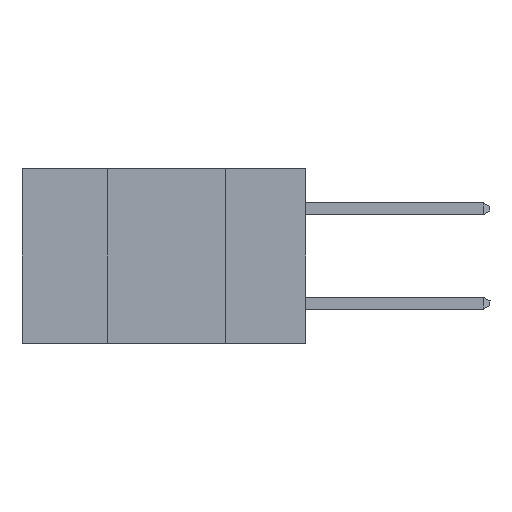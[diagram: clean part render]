
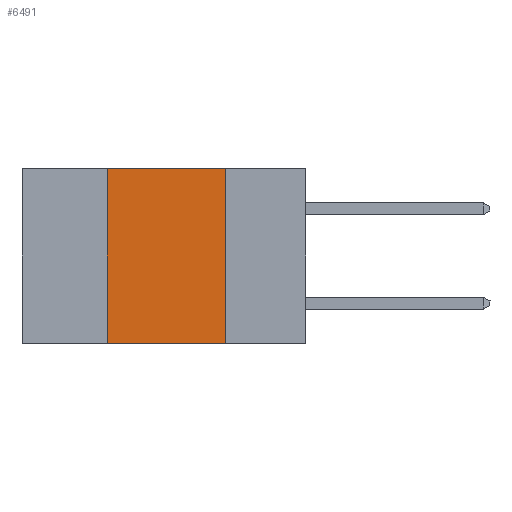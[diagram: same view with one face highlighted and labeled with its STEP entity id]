
A CAD part, left-side view. The second image highlights one B-rep face of the part: STEP entity #6491.
In plain terms, the highlighted planar face has unit normal (-1, 0, 0).
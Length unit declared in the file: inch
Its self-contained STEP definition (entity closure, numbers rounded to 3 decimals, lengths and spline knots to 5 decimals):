
#111 = VECTOR ( 'NONE', #6133, 39.37008 ) ;
#2327 = VECTOR ( 'NONE', #5412, 39.37008 ) ;
#3230 = LINE ( 'NONE', #7693, #8571 ) ;
#3792 = ORIENTED_EDGE ( 'NONE', *, *, #4248, .F. ) ;
#3851 = VERTEX_POINT ( 'NONE', #7272 ) ;
#3868 = ORIENTED_EDGE ( 'NONE', *, *, #4463, .F. ) ;
#4248 = EDGE_CURVE ( 'NONE', #3851, #10969, #10044, .T. ) ;
#4463 = EDGE_CURVE ( 'NONE', #10969, #12959, #3230, .T. ) ;
#5000 = EDGE_CURVE ( 'NONE', #13217, #12959, #14022, .T. ) ;
#5136 = CARTESIAN_POINT ( 'NONE',  ( 0., 0.6, 0. ) ) ;
#5210 = EDGE_CURVE ( 'NONE', #13217, #3851, #12426, .T. ) ;
#5412 = DIRECTION ( 'NONE',  ( 0., -1., 0. ) ) ;
#6133 = DIRECTION ( 'NONE',  ( 0., 0., 1. ) ) ;
#6328 = ORIENTED_EDGE ( 'NONE', *, *, #5000, .T. ) ;
#6337 = FACE_OUTER_BOUND ( 'NONE', #12297, .T. ) ;
#6429 = DIRECTION ( 'NONE',  ( 0., 0., -1. ) ) ;
#6491 = ADVANCED_FACE ( 'NONE', ( #6337 ), #8418, .F. ) ;
#6568 = DIRECTION ( 'NONE',  ( 0., 0., -1. ) ) ;
#6852 = CARTESIAN_POINT ( 'NONE',  ( 0., 0.17, -0.37 ) ) ;
#6956 = CARTESIAN_POINT ( 'NONE',  ( 0., 0.6, -0.37 ) ) ;
#7272 = CARTESIAN_POINT ( 'NONE',  ( 0., 0.42, 0. ) ) ;
#7686 = CARTESIAN_POINT ( 'NONE',  ( 0., 0.17, 0. ) ) ;
#7693 = CARTESIAN_POINT ( 'NONE',  ( 0., 0.17, 0. ) ) ;
#8418 = PLANE ( 'NONE',  #11963 ) ;
#8571 = VECTOR ( 'NONE', #6568, 39.37008 ) ;
#8695 = DIRECTION ( 'NONE',  ( 1., 0., 0. ) ) ;
#10044 = LINE ( 'NONE', #14464, #2327 ) ;
#10214 = CARTESIAN_POINT ( 'NONE',  ( 0., 0.42, -0.37 ) ) ;
#10809 = CARTESIAN_POINT ( 'NONE',  ( 0., 0.42, 0. ) ) ;
#10969 = VERTEX_POINT ( 'NONE', #7686 ) ;
#11022 = ORIENTED_EDGE ( 'NONE', *, *, #5210, .F. ) ;
#11735 = DIRECTION ( 'NONE',  ( 0., -1., 0. ) ) ;
#11963 = AXIS2_PLACEMENT_3D ( 'NONE', #5136, #8695, #6429 ) ;
#12043 = VECTOR ( 'NONE', #11735, 39.37008 ) ;
#12297 = EDGE_LOOP ( 'NONE', ( #3868, #3792, #11022, #6328 ) ) ;
#12426 = LINE ( 'NONE', #10809, #111 ) ;
#12959 = VERTEX_POINT ( 'NONE', #6852 ) ;
#13217 = VERTEX_POINT ( 'NONE', #10214 ) ;
#14022 = LINE ( 'NONE', #6956, #12043 ) ;
#14464 = CARTESIAN_POINT ( 'NONE',  ( 0., 0.6, 0. ) ) ;
